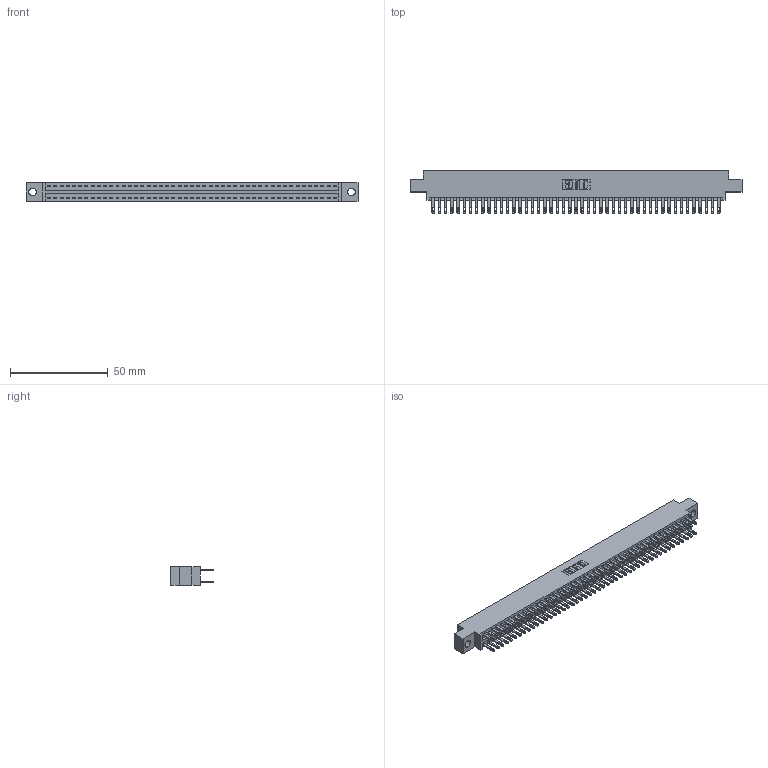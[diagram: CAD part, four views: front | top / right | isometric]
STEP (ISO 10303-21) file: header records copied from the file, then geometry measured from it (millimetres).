
FILE_DESCRIPTION (( 'STEP AP203' ), '1' );
FILE_NAME ('346-094-500-804.STEP', '2022-05-26T09:10:34', ( '' ), ( '' ), 'SwSTEP 2.0', 'SolidWorks 2020', '' );
FILE_SCHEMA (( 'CONFIG_CONTROL_DESIGN' ));
Length unit declared in the file: inch
Products named in the file (3): 345-292-001_345-293-100; 346 Part_0.170 Offset - 0.156 Dia-TH; 346-094-500-804
Assembly tree (95 placements, depth 2):
  346-094-500-804
    346 Part_0.170 Offset - 0.156 Dia-TH
    345-292-001_345-293-100  x94
Bounding box: 169.8 x 21.84 x 9.4 mm (x, y, z)
Volume: 16623 mm3; surface area: 23939.4 mm2
Topology: 95 solids, 95 shells, 4652 faces, 14195 edges, 9462 vertices
Faces by surface type: plane 2820, cylinder 1832
Entity records: 30481 total; most frequent: CARTESIAN_POINT 5022, ORIENTED_EDGE 4954, DIRECTION 4477, EDGE_CURVE 2477, VECTOR 2153, LINE 2153, VERTEX_POINT 1650, AXIS2_PLACEMENT_3D 1162
